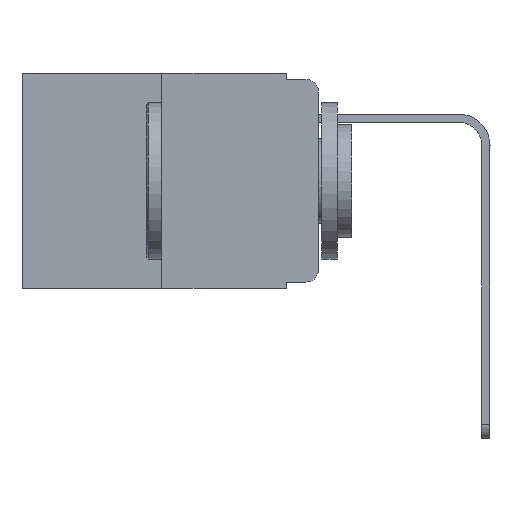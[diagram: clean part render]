
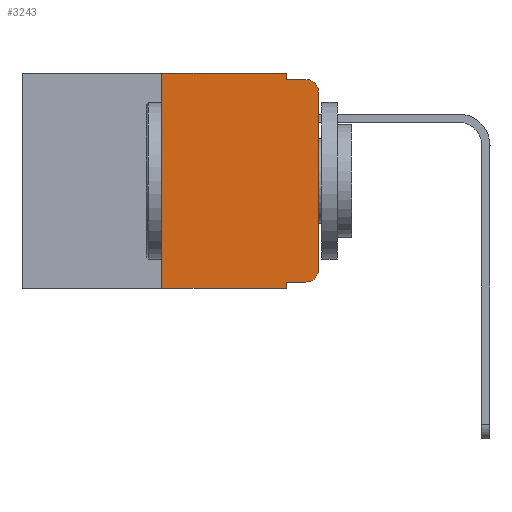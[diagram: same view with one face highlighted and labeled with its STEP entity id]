
A CAD part, left-side view. The second image highlights one B-rep face of the part: STEP entity #3243.
In plain terms, the highlighted planar face has unit normal (-1, 0, 0).
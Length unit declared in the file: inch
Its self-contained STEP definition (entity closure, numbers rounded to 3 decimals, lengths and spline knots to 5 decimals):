
#74 = DIRECTION ( 'NONE',  ( 0., 0., 1. ) ) ;
#437 = VECTOR ( 'NONE', #11635, 39.37008 ) ;
#583 = DIRECTION ( 'NONE',  ( 0., 0., -1. ) ) ;
#585 = LINE ( 'NONE', #23177, #22004 ) ;
#705 = CARTESIAN_POINT ( 'NONE',  ( 0., 0., -0.03 ) ) ;
#848 = DIRECTION ( 'NONE',  ( 0., -1., 0. ) ) ;
#966 = VECTOR ( 'NONE', #74, 39.37008 ) ;
#2052 = CARTESIAN_POINT ( 'NONE',  ( 0., 0.051, 0. ) ) ;
#2416 = LINE ( 'NONE', #15728, #13441 ) ;
#2694 = ORIENTED_EDGE ( 'NONE', *, *, #7688, .F. ) ;
#3114 = CARTESIAN_POINT ( 'NONE',  ( 0., 0.051, 0. ) ) ;
#3243 = ADVANCED_FACE ( 'NONE', ( #16814 ), #22002, .F. ) ;
#3281 = ORIENTED_EDGE ( 'NONE', *, *, #9651, .T. ) ;
#3729 = CARTESIAN_POINT ( 'NONE',  ( 0., 0.473, -0.343 ) ) ;
#3746 = CARTESIAN_POINT ( 'NONE',  ( 0., 0.02, -0.01 ) ) ;
#3988 = DIRECTION ( 'NONE',  ( 0., 0., -1. ) ) ;
#4053 = EDGE_CURVE ( 'NONE', #20172, #18024, #8675, .T. ) ;
#4740 = LINE ( 'NONE', #23766, #966 ) ;
#4742 = VERTEX_POINT ( 'NONE', #23845 ) ;
#4752 = EDGE_CURVE ( 'NONE', #4742, #18024, #11850, .T. ) ;
#4949 = CARTESIAN_POINT ( 'NONE',  ( 0., 0.25, -0.343 ) ) ;
#5066 = LINE ( 'NONE', #22366, #437 ) ;
#5175 = VECTOR ( 'NONE', #18340, 39.37008 ) ;
#6029 = CARTESIAN_POINT ( 'NONE',  ( 0., 0.02, -0.03 ) ) ;
#6577 = CARTESIAN_POINT ( 'NONE',  ( 0., 0.25, 0. ) ) ;
#6773 = VECTOR ( 'NONE', #11690, 39.37008 ) ;
#7119 = ORIENTED_EDGE ( 'NONE', *, *, #22956, .T. ) ;
#7155 = CARTESIAN_POINT ( 'NONE',  ( 0., 0.02, -0.313 ) ) ;
#7411 = VERTEX_POINT ( 'NONE', #2052 ) ;
#7688 = EDGE_CURVE ( 'NONE', #14959, #7411, #2416, .T. ) ;
#8486 = EDGE_LOOP ( 'NONE', ( #3281, #20155, #8812, #14420, #2694, #11433, #21754, #15400, #22044, #7119 ) ) ;
#8675 = LINE ( 'NONE', #3729, #19071 ) ;
#8812 = ORIENTED_EDGE ( 'NONE', *, *, #22267, .F. ) ;
#9037 = DIRECTION ( 'NONE',  ( 0., 0., -1. ) ) ;
#9106 = LINE ( 'NONE', #15303, #6773 ) ;
#9263 = CIRCLE ( 'NONE', #18599, 0.02 ) ;
#9399 = EDGE_CURVE ( 'NONE', #4742, #21147, #5066, .T. ) ;
#9651 = EDGE_CURVE ( 'NONE', #20491, #22241, #9106, .T. ) ;
#10041 = EDGE_CURVE ( 'NONE', #20172, #14959, #4740, .T. ) ;
#10962 = CARTESIAN_POINT ( 'NONE',  ( 0., 0.473, 0. ) ) ;
#11232 = VERTEX_POINT ( 'NONE', #3746 ) ;
#11433 = ORIENTED_EDGE ( 'NONE', *, *, #10041, .F. ) ;
#11601 = DIRECTION ( 'NONE',  ( 1., 0., 0. ) ) ;
#11635 = DIRECTION ( 'NONE',  ( 0., -1., 0. ) ) ;
#11690 = DIRECTION ( 'NONE',  ( 0., 0., 1. ) ) ;
#11850 = LINE ( 'NONE', #14628, #5175 ) ;
#12415 = CARTESIAN_POINT ( 'NONE',  ( 0., 0.02, -0.333 ) ) ;
#12499 = DIRECTION ( 'NONE',  ( 0., 0., -1. ) ) ;
#13356 = CARTESIAN_POINT ( 'NONE',  ( 0., 0.051, -0.01 ) ) ;
#13441 = VECTOR ( 'NONE', #848, 39.37008 ) ;
#13598 = VERTEX_POINT ( 'NONE', #13356 ) ;
#13979 = DIRECTION ( 'NONE',  ( 0., -1., 0. ) ) ;
#14420 = ORIENTED_EDGE ( 'NONE', *, *, #22512, .F. ) ;
#14628 = CARTESIAN_POINT ( 'NONE',  ( 0., 0.051, 0. ) ) ;
#14756 = EDGE_CURVE ( 'NONE', #22241, #11232, #22096, .T. ) ;
#14959 = VERTEX_POINT ( 'NONE', #6577 ) ;
#15303 = CARTESIAN_POINT ( 'NONE',  ( 0., 0., 0. ) ) ;
#15400 = ORIENTED_EDGE ( 'NONE', *, *, #4752, .F. ) ;
#15531 = AXIS2_PLACEMENT_3D ( 'NONE', #10962, #11601, #3988 ) ;
#15728 = CARTESIAN_POINT ( 'NONE',  ( 0., 0.473, 0. ) ) ;
#16441 = DIRECTION ( 'NONE',  ( 0., -1., 0. ) ) ;
#16454 = DIRECTION ( 'NONE',  ( -1., 0., 0. ) ) ;
#16488 = LINE ( 'NONE', #3114, #20523 ) ;
#16814 = FACE_OUTER_BOUND ( 'NONE', #8486, .T. ) ;
#17014 = DIRECTION ( 'NONE',  ( -1., 0., 0. ) ) ;
#18024 = VERTEX_POINT ( 'NONE', #18443 ) ;
#18340 = DIRECTION ( 'NONE',  ( 0., 0., -1. ) ) ;
#18443 = CARTESIAN_POINT ( 'NONE',  ( 0., 0.051, -0.343 ) ) ;
#18599 = AXIS2_PLACEMENT_3D ( 'NONE', #7155, #16454, #12499 ) ;
#19071 = VECTOR ( 'NONE', #16441, 39.37008 ) ;
#20155 = ORIENTED_EDGE ( 'NONE', *, *, #14756, .T. ) ;
#20172 = VERTEX_POINT ( 'NONE', #4949 ) ;
#20491 = VERTEX_POINT ( 'NONE', #22552 ) ;
#20523 = VECTOR ( 'NONE', #9037, 39.37008 ) ;
#21147 = VERTEX_POINT ( 'NONE', #12415 ) ;
#21754 = ORIENTED_EDGE ( 'NONE', *, *, #4053, .T. ) ;
#22002 = PLANE ( 'NONE',  #15531 ) ;
#22004 = VECTOR ( 'NONE', #13979, 39.37008 ) ;
#22044 = ORIENTED_EDGE ( 'NONE', *, *, #9399, .T. ) ;
#22096 = CIRCLE ( 'NONE', #22822, 0.02 ) ;
#22241 = VERTEX_POINT ( 'NONE', #705 ) ;
#22267 = EDGE_CURVE ( 'NONE', #13598, #11232, #585, .T. ) ;
#22366 = CARTESIAN_POINT ( 'NONE',  ( 0., 0.051, -0.333 ) ) ;
#22512 = EDGE_CURVE ( 'NONE', #7411, #13598, #16488, .T. ) ;
#22552 = CARTESIAN_POINT ( 'NONE',  ( 0., 0., -0.313 ) ) ;
#22822 = AXIS2_PLACEMENT_3D ( 'NONE', #6029, #17014, #583 ) ;
#22956 = EDGE_CURVE ( 'NONE', #21147, #20491, #9263, .T. ) ;
#23177 = CARTESIAN_POINT ( 'NONE',  ( 0., 0.051, -0.01 ) ) ;
#23766 = CARTESIAN_POINT ( 'NONE',  ( 0., 0.25, 0. ) ) ;
#23845 = CARTESIAN_POINT ( 'NONE',  ( 0., 0.051, -0.333 ) ) ;
